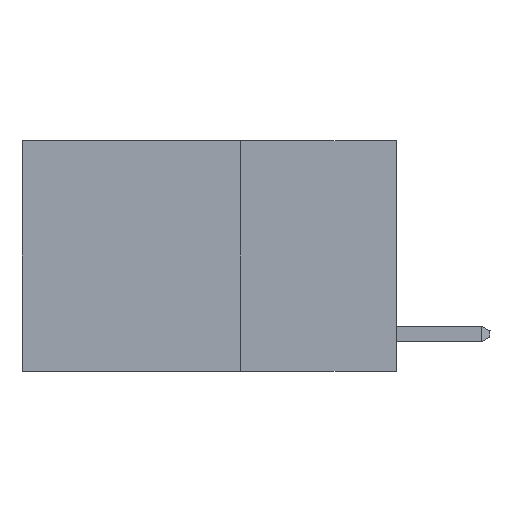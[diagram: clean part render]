
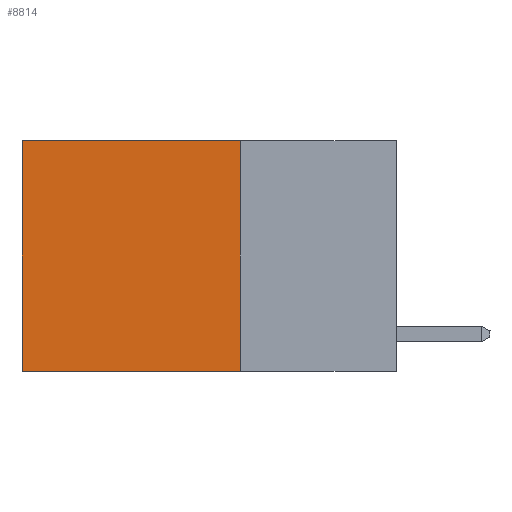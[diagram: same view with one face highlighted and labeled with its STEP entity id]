
A CAD part, left-side view. The second image highlights one B-rep face of the part: STEP entity #8814.
In plain terms, the highlighted planar face has unit normal (-1, 0, 0).
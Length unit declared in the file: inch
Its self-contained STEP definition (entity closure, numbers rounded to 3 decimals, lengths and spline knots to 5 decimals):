
#528 = CARTESIAN_POINT ( 'NONE',  ( 0.2625, 0.25, 0. ) ) ;
#561 = VECTOR ( 'NONE', #8266, 39.37008 ) ;
#1776 = CARTESIAN_POINT ( 'NONE',  ( 0.2625, 0.25, -0.37 ) ) ;
#2486 = EDGE_LOOP ( 'NONE', ( #5009, #6184, #12711, #11393 ) ) ;
#3109 = VECTOR ( 'NONE', #13247, 39.37008 ) ;
#3433 = LINE ( 'NONE', #5565, #17033 ) ;
#4442 = LINE ( 'NONE', #8397, #561 ) ;
#5009 = ORIENTED_EDGE ( 'NONE', *, *, #8856, .T. ) ;
#5393 = EDGE_CURVE ( 'NONE', #10246, #6472, #8304, .T. ) ;
#5565 = CARTESIAN_POINT ( 'NONE',  ( 0.2625, 0.25, -0.37 ) ) ;
#5772 = DIRECTION ( 'NONE',  ( 1., 0., 0. ) ) ;
#6184 = ORIENTED_EDGE ( 'NONE', *, *, #15539, .F. ) ;
#6472 = VERTEX_POINT ( 'NONE', #7777 ) ;
#7777 = CARTESIAN_POINT ( 'NONE',  ( 0.2625, 0.6, 0. ) ) ;
#8188 = DIRECTION ( 'NONE',  ( 0., 1., 0. ) ) ;
#8266 = DIRECTION ( 'NONE',  ( 0., 0., -1. ) ) ;
#8304 = LINE ( 'NONE', #16057, #13580 ) ;
#8397 = CARTESIAN_POINT ( 'NONE',  ( 0.2625, 0.25, 0. ) ) ;
#8814 = ADVANCED_FACE ( 'NONE', ( #16844 ), #13125, .F. ) ;
#8856 = EDGE_CURVE ( 'NONE', #6472, #9249, #18759, .T. ) ;
#9249 = VERTEX_POINT ( 'NONE', #17208 ) ;
#10246 = VERTEX_POINT ( 'NONE', #528 ) ;
#10731 = EDGE_CURVE ( 'NONE', #10246, #10833, #4442, .T. ) ;
#10833 = VERTEX_POINT ( 'NONE', #1776 ) ;
#11007 = AXIS2_PLACEMENT_3D ( 'NONE', #11602, #5772, #11735 ) ;
#11393 = ORIENTED_EDGE ( 'NONE', *, *, #5393, .T. ) ;
#11602 = CARTESIAN_POINT ( 'NONE',  ( 0.2625, 0.25, 0. ) ) ;
#11735 = DIRECTION ( 'NONE',  ( 0., 0., -1. ) ) ;
#11809 = CARTESIAN_POINT ( 'NONE',  ( 0.2625, 0.6, 0. ) ) ;
#12711 = ORIENTED_EDGE ( 'NONE', *, *, #10731, .F. ) ;
#13125 = PLANE ( 'NONE',  #11007 ) ;
#13247 = DIRECTION ( 'NONE',  ( 0., 0., -1. ) ) ;
#13580 = VECTOR ( 'NONE', #17519, 39.37008 ) ;
#15539 = EDGE_CURVE ( 'NONE', #10833, #9249, #3433, .T. ) ;
#16057 = CARTESIAN_POINT ( 'NONE',  ( 0.2625, 0.25, 0. ) ) ;
#16844 = FACE_OUTER_BOUND ( 'NONE', #2486, .T. ) ;
#17033 = VECTOR ( 'NONE', #8188, 39.37008 ) ;
#17208 = CARTESIAN_POINT ( 'NONE',  ( 0.2625, 0.6, -0.37 ) ) ;
#17519 = DIRECTION ( 'NONE',  ( 0., 1., 0. ) ) ;
#18759 = LINE ( 'NONE', #11809, #3109 ) ;
